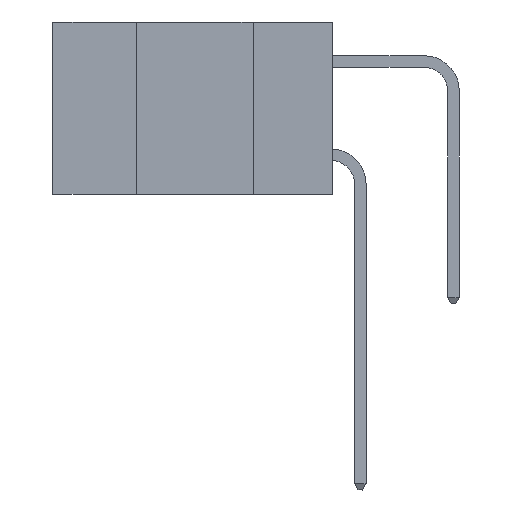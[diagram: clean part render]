
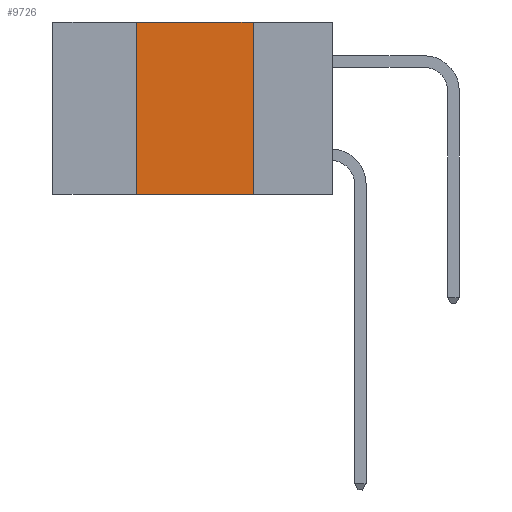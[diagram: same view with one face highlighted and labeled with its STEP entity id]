
A CAD part, left-side view. The second image highlights one B-rep face of the part: STEP entity #9726.
In plain terms, the highlighted planar face has unit normal (-1, 0, 0).
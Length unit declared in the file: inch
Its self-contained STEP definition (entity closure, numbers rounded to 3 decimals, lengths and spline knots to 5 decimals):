
#289 = ORIENTED_EDGE ( 'NONE', *, *, #25084, .T. ) ;
#1165 = PLANE ( 'NONE',  #17919 ) ;
#3807 = VERTEX_POINT ( 'NONE', #7389 ) ;
#4002 = CARTESIAN_POINT ( 'NONE',  ( 0., 0.6, 0. ) ) ;
#6491 = EDGE_LOOP ( 'NONE', ( #29115, #27007, #12515, #289 ) ) ;
#6840 = DIRECTION ( 'NONE',  ( 1., 0., 0. ) ) ;
#7389 = CARTESIAN_POINT ( 'NONE',  ( 0., 0.42, -0.37 ) ) ;
#8756 = CARTESIAN_POINT ( 'NONE',  ( 0., 0.42, 0. ) ) ;
#9726 = ADVANCED_FACE ( 'NONE', ( #20445 ), #1165, .F. ) ;
#10588 = CARTESIAN_POINT ( 'NONE',  ( 0., 0.6, 0. ) ) ;
#11331 = LINE ( 'NONE', #12250, #20298 ) ;
#12115 = CARTESIAN_POINT ( 'NONE',  ( 0., 0.17, 0. ) ) ;
#12150 = VERTEX_POINT ( 'NONE', #8756 ) ;
#12250 = CARTESIAN_POINT ( 'NONE',  ( 0., 0.42, 0. ) ) ;
#12319 = CARTESIAN_POINT ( 'NONE',  ( 0., 0.17, 0. ) ) ;
#12321 = EDGE_CURVE ( 'NONE', #3807, #12150, #11331, .T. ) ;
#12515 = ORIENTED_EDGE ( 'NONE', *, *, #12321, .F. ) ;
#13643 = VERTEX_POINT ( 'NONE', #34572 ) ;
#14801 = LINE ( 'NONE', #12115, #28486 ) ;
#14844 = DIRECTION ( 'NONE',  ( 0., 0., -1. ) ) ;
#15924 = DIRECTION ( 'NONE',  ( 0., -1., 0. ) ) ;
#17765 = EDGE_CURVE ( 'NONE', #25627, #13643, #14801, .T. ) ;
#17793 = CARTESIAN_POINT ( 'NONE',  ( 0., 0.6, -0.37 ) ) ;
#17919 = AXIS2_PLACEMENT_3D ( 'NONE', #4002, #6840, #25975 ) ;
#20298 = VECTOR ( 'NONE', #20425, 39.37008 ) ;
#20425 = DIRECTION ( 'NONE',  ( 0., 0., 1. ) ) ;
#20445 = FACE_OUTER_BOUND ( 'NONE', #6491, .T. ) ;
#20514 = DIRECTION ( 'NONE',  ( 0., -1., 0. ) ) ;
#25084 = EDGE_CURVE ( 'NONE', #3807, #13643, #25127, .T. ) ;
#25127 = LINE ( 'NONE', #17793, #31630 ) ;
#25627 = VERTEX_POINT ( 'NONE', #12319 ) ;
#25975 = DIRECTION ( 'NONE',  ( 0., 0., -1. ) ) ;
#26935 = VECTOR ( 'NONE', #15924, 39.37008 ) ;
#27007 = ORIENTED_EDGE ( 'NONE', *, *, #27098, .F. ) ;
#27098 = EDGE_CURVE ( 'NONE', #12150, #25627, #34275, .T. ) ;
#28486 = VECTOR ( 'NONE', #14844, 39.37008 ) ;
#29115 = ORIENTED_EDGE ( 'NONE', *, *, #17765, .F. ) ;
#31630 = VECTOR ( 'NONE', #20514, 39.37008 ) ;
#34275 = LINE ( 'NONE', #10588, #26935 ) ;
#34572 = CARTESIAN_POINT ( 'NONE',  ( 0., 0.17, -0.37 ) ) ;
